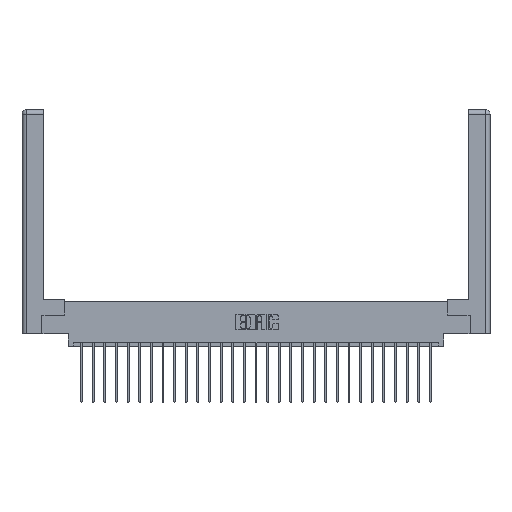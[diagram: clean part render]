
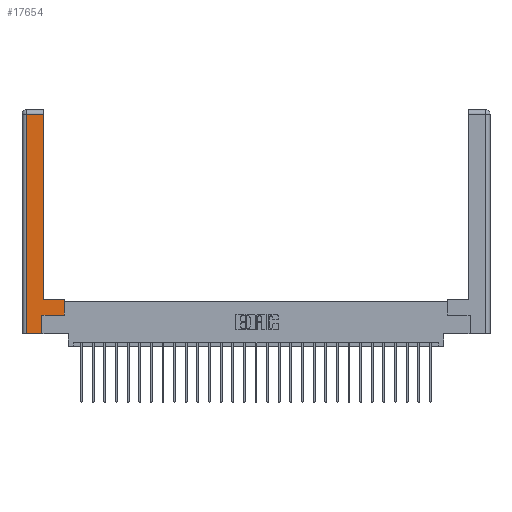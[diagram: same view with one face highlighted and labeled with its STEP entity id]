
A CAD part, top view. The second image highlights one B-rep face of the part: STEP entity #17654.
In plain terms, the highlighted planar face has unit normal (0, 0, 1).
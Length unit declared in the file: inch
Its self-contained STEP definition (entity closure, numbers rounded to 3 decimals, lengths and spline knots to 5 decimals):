
#56 = EDGE_CURVE ( 'NONE', #2957, #22034, #1063, .T. ) ;
#299 = DIRECTION ( 'NONE',  ( -1., 0., 0. ) ) ;
#311 = PLANE ( 'NONE',  #12536 ) ;
#431 = DIRECTION ( 'NONE',  ( -1., 0., 0. ) ) ;
#997 = CARTESIAN_POINT ( 'NONE',  ( 0.295, 0.45, 0. ) ) ;
#1028 = ORIENTED_EDGE ( 'NONE', *, *, #15772, .T. ) ;
#1063 = LINE ( 'NONE', #19064, #17114 ) ;
#1602 = LINE ( 'NONE', #5723, #9820 ) ;
#1904 = CARTESIAN_POINT ( 'NONE',  ( 0.265, 0., 0. ) ) ;
#2957 = VERTEX_POINT ( 'NONE', #24523 ) ;
#3048 = ORIENTED_EDGE ( 'NONE', *, *, #19701, .T. ) ;
#4027 = DIRECTION ( 'NONE',  ( 1., 0., 0. ) ) ;
#4034 = LINE ( 'NONE', #15622, #20808 ) ;
#4911 = EDGE_LOOP ( 'NONE', ( #13981, #3048, #10705, #22385, #25647, #1028, #18368, #16970 ) ) ;
#5181 = LINE ( 'NONE', #11156, #21219 ) ;
#5723 = CARTESIAN_POINT ( 'NONE',  ( 0.265, 0.245, 0. ) ) ;
#5984 = DIRECTION ( 'NONE',  ( 0., 1., 0. ) ) ;
#6905 = VERTEX_POINT ( 'NONE', #8043 ) ;
#7106 = LINE ( 'NONE', #24173, #15664 ) ;
#8043 = CARTESIAN_POINT ( 'NONE',  ( 0.295, 2.94, 0. ) ) ;
#8905 = EDGE_CURVE ( 'NONE', #8991, #6905, #4034, .T. ) ;
#8991 = VERTEX_POINT ( 'NONE', #997 ) ;
#9120 = DIRECTION ( 'NONE',  ( 0., 1., 0. ) ) ;
#9495 = VERTEX_POINT ( 'NONE', #22366 ) ;
#9820 = VECTOR ( 'NONE', #14588, 39.37008 ) ;
#10108 = VERTEX_POINT ( 'NONE', #20982 ) ;
#10705 = ORIENTED_EDGE ( 'NONE', *, *, #18025, .T. ) ;
#11156 = CARTESIAN_POINT ( 'NONE',  ( 0.0615, 2.94, 0. ) ) ;
#11696 = EDGE_CURVE ( 'NONE', #10108, #18689, #1602, .T. ) ;
#11958 = VECTOR ( 'NONE', #21609, 39.37008 ) ;
#12536 = AXIS2_PLACEMENT_3D ( 'NONE', #22181, #20275, #20165 ) ;
#13717 = LINE ( 'NONE', #19540, #17133 ) ;
#13981 = ORIENTED_EDGE ( 'NONE', *, *, #8905, .T. ) ;
#14588 = DIRECTION ( 'NONE',  ( 0., 1., 0. ) ) ;
#15332 = VERTEX_POINT ( 'NONE', #15908 ) ;
#15515 = EDGE_CURVE ( 'NONE', #22034, #8991, #7106, .T. ) ;
#15622 = CARTESIAN_POINT ( 'NONE',  ( 0.295, 3., 0. ) ) ;
#15664 = VECTOR ( 'NONE', #431, 39.37008 ) ;
#15772 = EDGE_CURVE ( 'NONE', #18689, #2957, #23815, .T. ) ;
#15797 = FACE_OUTER_BOUND ( 'NONE', #4911, .T. ) ;
#15908 = CARTESIAN_POINT ( 'NONE',  ( 0.0615, 0., 0. ) ) ;
#16970 = ORIENTED_EDGE ( 'NONE', *, *, #15515, .T. ) ;
#17114 = VECTOR ( 'NONE', #5984, 39.37008 ) ;
#17133 = VECTOR ( 'NONE', #20229, 39.37008 ) ;
#17654 = ADVANCED_FACE ( 'NONE', ( #15797 ), #311, .F. ) ;
#17767 = LINE ( 'NONE', #1904, #11958 ) ;
#18025 = EDGE_CURVE ( 'NONE', #9495, #15332, #13717, .T. ) ;
#18368 = ORIENTED_EDGE ( 'NONE', *, *, #56, .T. ) ;
#18689 = VERTEX_POINT ( 'NONE', #25047 ) ;
#18771 = EDGE_CURVE ( 'NONE', #15332, #10108, #17767, .T. ) ;
#19064 = CARTESIAN_POINT ( 'NONE',  ( 0.565, 0.45, 0. ) ) ;
#19540 = CARTESIAN_POINT ( 'NONE',  ( 0.0615, 0., 0. ) ) ;
#19701 = EDGE_CURVE ( 'NONE', #6905, #9495, #5181, .T. ) ;
#20165 = DIRECTION ( 'NONE',  ( -1., 0., 0. ) ) ;
#20229 = DIRECTION ( 'NONE',  ( 0., -1., 0. ) ) ;
#20275 = DIRECTION ( 'NONE',  ( 0., 0., -1. ) ) ;
#20808 = VECTOR ( 'NONE', #9120, 39.37008 ) ;
#20982 = CARTESIAN_POINT ( 'NONE',  ( 0.265, 0., 0. ) ) ;
#21219 = VECTOR ( 'NONE', #299, 39.37008 ) ;
#21452 = VECTOR ( 'NONE', #4027, 39.37008 ) ;
#21609 = DIRECTION ( 'NONE',  ( 1., 0., 0. ) ) ;
#22034 = VERTEX_POINT ( 'NONE', #23634 ) ;
#22181 = CARTESIAN_POINT ( 'NONE',  ( 0., 0., 0. ) ) ;
#22366 = CARTESIAN_POINT ( 'NONE',  ( 0.0615, 2.94, 0. ) ) ;
#22385 = ORIENTED_EDGE ( 'NONE', *, *, #18771, .T. ) ;
#23634 = CARTESIAN_POINT ( 'NONE',  ( 0.565, 0.45, 0. ) ) ;
#23815 = LINE ( 'NONE', #28175, #21452 ) ;
#24173 = CARTESIAN_POINT ( 'NONE',  ( 0.295, 0.45, 0. ) ) ;
#24523 = CARTESIAN_POINT ( 'NONE',  ( 0.565, 0.245, 0. ) ) ;
#25047 = CARTESIAN_POINT ( 'NONE',  ( 0.265, 0.245, 0. ) ) ;
#25647 = ORIENTED_EDGE ( 'NONE', *, *, #11696, .T. ) ;
#28175 = CARTESIAN_POINT ( 'NONE',  ( 0.565, 0.245, 0. ) ) ;
